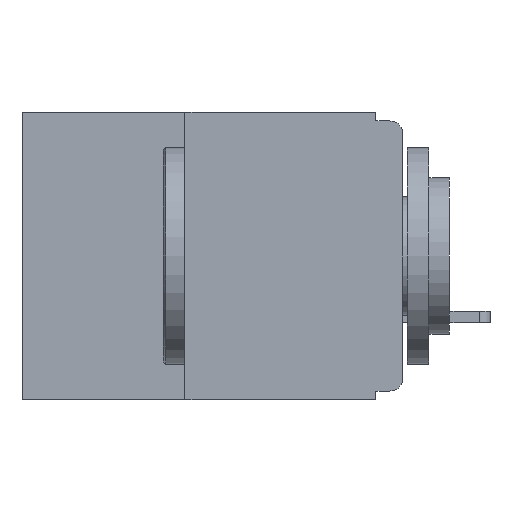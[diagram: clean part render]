
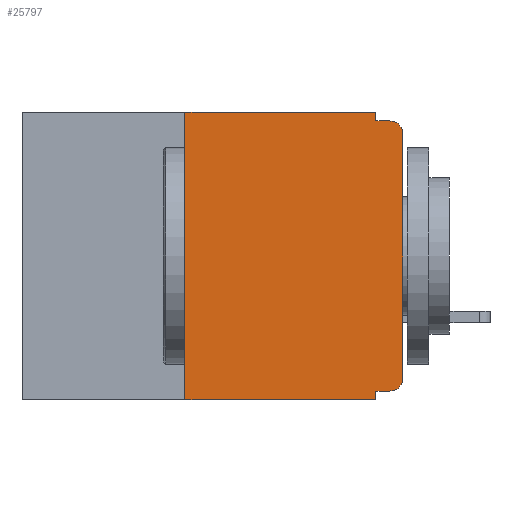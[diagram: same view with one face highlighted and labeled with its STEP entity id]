
A CAD part, left-side view. The second image highlights one B-rep face of the part: STEP entity #25797.
In plain terms, the highlighted planar face has unit normal (-1, 0, 0).
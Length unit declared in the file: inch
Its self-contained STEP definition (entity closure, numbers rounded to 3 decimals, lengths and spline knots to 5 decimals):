
#23 = CARTESIAN_POINT ( 'NONE',  ( 0., 0., -0.32 ) ) ;
#103 = DIRECTION ( 'NONE',  ( 0., -1., 0. ) ) ;
#634 = DIRECTION ( 'NONE',  ( 0., 0., -1. ) ) ;
#754 = FACE_OUTER_BOUND ( 'NONE', #24668, .T. ) ;
#768 = AXIS2_PLACEMENT_3D ( 'NONE', #10609, #28181, #13141 ) ;
#1409 = CARTESIAN_POINT ( 'NONE',  ( 0., 0.25, -0.33 ) ) ;
#1519 = ORIENTED_EDGE ( 'NONE', *, *, #18373, .F. ) ;
#1809 = CARTESIAN_POINT ( 'NONE',  ( 0., 0.031, 0. ) ) ;
#2441 = CARTESIAN_POINT ( 'NONE',  ( 0., 0.031, -0.33 ) ) ;
#2605 = PLANE ( 'NONE',  #13702 ) ;
#3797 = CARTESIAN_POINT ( 'NONE',  ( 0., 0.437, -0.33 ) ) ;
#4148 = VECTOR ( 'NONE', #22255, 39.37008 ) ;
#4818 = VERTEX_POINT ( 'NONE', #17904 ) ;
#5098 = LINE ( 'NONE', #14579, #24452 ) ;
#5212 = EDGE_CURVE ( 'NONE', #6871, #4818, #26192, .T. ) ;
#5271 = CARTESIAN_POINT ( 'NONE',  ( 0., 0.437, 0. ) ) ;
#5779 = LINE ( 'NONE', #1809, #4148 ) ;
#6827 = VERTEX_POINT ( 'NONE', #25525 ) ;
#6871 = VERTEX_POINT ( 'NONE', #13091 ) ;
#6910 = ORIENTED_EDGE ( 'NONE', *, *, #32550, .F. ) ;
#7882 = DIRECTION ( 'NONE',  ( 0., 0., -1. ) ) ;
#8579 = LINE ( 'NONE', #3797, #21163 ) ;
#8586 = VERTEX_POINT ( 'NONE', #2441 ) ;
#9328 = EDGE_CURVE ( 'NONE', #19104, #8586, #8579, .T. ) ;
#9631 = ORIENTED_EDGE ( 'NONE', *, *, #24382, .F. ) ;
#10068 = VECTOR ( 'NONE', #15318, 39.37008 ) ;
#10439 = ORIENTED_EDGE ( 'NONE', *, *, #27580, .F. ) ;
#10609 = CARTESIAN_POINT ( 'NONE',  ( 0., 0.015, -0.305 ) ) ;
#10892 = VERTEX_POINT ( 'NONE', #25152 ) ;
#10914 = LINE ( 'NONE', #23, #32439 ) ;
#11110 = VECTOR ( 'NONE', #103, 39.37008 ) ;
#11648 = DIRECTION ( 'NONE',  ( 0., 0., 1. ) ) ;
#12910 = CIRCLE ( 'NONE', #768, 0.015 ) ;
#13091 = CARTESIAN_POINT ( 'NONE',  ( 0., 0., -0.305 ) ) ;
#13141 = DIRECTION ( 'NONE',  ( 0., 0., -1. ) ) ;
#13702 = AXIS2_PLACEMENT_3D ( 'NONE', #5271, #22924, #7882 ) ;
#13821 = ORIENTED_EDGE ( 'NONE', *, *, #16783, .F. ) ;
#14011 = CARTESIAN_POINT ( 'NONE',  ( 0., 0.25, 0. ) ) ;
#14579 = CARTESIAN_POINT ( 'NONE',  ( 0., 0., -0.01 ) ) ;
#14697 = LINE ( 'NONE', #1409, #28028 ) ;
#15318 = DIRECTION ( 'NONE',  ( 0., 0., -1. ) ) ;
#16006 = DIRECTION ( 'NONE',  ( -1., 0., 0. ) ) ;
#16510 = VERTEX_POINT ( 'NONE', #14011 ) ;
#16783 = EDGE_CURVE ( 'NONE', #17514, #8586, #21857, .T. ) ;
#17514 = VERTEX_POINT ( 'NONE', #28196 ) ;
#17852 = LINE ( 'NONE', #18043, #11110 ) ;
#17904 = CARTESIAN_POINT ( 'NONE',  ( 0., 0., -0.025 ) ) ;
#17944 = CARTESIAN_POINT ( 'NONE',  ( 0., 0.25, -0.33 ) ) ;
#17963 = DIRECTION ( 'NONE',  ( 0., 1., 0. ) ) ;
#18043 = CARTESIAN_POINT ( 'NONE',  ( 0., 0.437, 0. ) ) ;
#18373 = EDGE_CURVE ( 'NONE', #19104, #16510, #14697, .T. ) ;
#19019 = DIRECTION ( 'NONE',  ( 0., -1., 0. ) ) ;
#19104 = VERTEX_POINT ( 'NONE', #17944 ) ;
#19611 = DIRECTION ( 'NONE',  ( 0., -1., 0. ) ) ;
#19684 = VERTEX_POINT ( 'NONE', #30311 ) ;
#20657 = VERTEX_POINT ( 'NONE', #25388 ) ;
#21163 = VECTOR ( 'NONE', #19019, 39.37008 ) ;
#21264 = ORIENTED_EDGE ( 'NONE', *, *, #9328, .T. ) ;
#21857 = LINE ( 'NONE', #30287, #10068 ) ;
#22099 = ORIENTED_EDGE ( 'NONE', *, *, #5212, .T. ) ;
#22110 = CIRCLE ( 'NONE', #29321, 0.015 ) ;
#22255 = DIRECTION ( 'NONE',  ( 0., 0., -1. ) ) ;
#22924 = DIRECTION ( 'NONE',  ( 1., 0., 0. ) ) ;
#24382 = EDGE_CURVE ( 'NONE', #6827, #10892, #5779, .T. ) ;
#24452 = VECTOR ( 'NONE', #19611, 39.37008 ) ;
#24493 = CARTESIAN_POINT ( 'NONE',  ( 0., 0., 0. ) ) ;
#24612 = DIRECTION ( 'NONE',  ( 0., 0., 1. ) ) ;
#24622 = EDGE_CURVE ( 'NONE', #20657, #6871, #12910, .T. ) ;
#24668 = EDGE_LOOP ( 'NONE', ( #22099, #32067, #25382, #9631, #10439, #1519, #21264, #13821, #6910, #27965 ) ) ;
#25152 = CARTESIAN_POINT ( 'NONE',  ( 0., 0.031, -0.01 ) ) ;
#25382 = ORIENTED_EDGE ( 'NONE', *, *, #28004, .F. ) ;
#25388 = CARTESIAN_POINT ( 'NONE',  ( 0., 0.015, -0.32 ) ) ;
#25525 = CARTESIAN_POINT ( 'NONE',  ( 0., 0.031, 0. ) ) ;
#25797 = ADVANCED_FACE ( 'NONE', ( #754 ), #2605, .F. ) ;
#26192 = LINE ( 'NONE', #24493, #31964 ) ;
#27580 = EDGE_CURVE ( 'NONE', #16510, #6827, #17852, .T. ) ;
#27965 = ORIENTED_EDGE ( 'NONE', *, *, #24622, .T. ) ;
#28004 = EDGE_CURVE ( 'NONE', #10892, #19684, #5098, .T. ) ;
#28028 = VECTOR ( 'NONE', #11648, 39.37008 ) ;
#28181 = DIRECTION ( 'NONE',  ( -1., 0., 0. ) ) ;
#28196 = CARTESIAN_POINT ( 'NONE',  ( 0., 0.031, -0.32 ) ) ;
#28321 = EDGE_CURVE ( 'NONE', #4818, #19684, #22110, .T. ) ;
#29321 = AXIS2_PLACEMENT_3D ( 'NONE', #30956, #16006, #634 ) ;
#30287 = CARTESIAN_POINT ( 'NONE',  ( 0., 0.031, -0.33 ) ) ;
#30311 = CARTESIAN_POINT ( 'NONE',  ( 0., 0.015, -0.01 ) ) ;
#30956 = CARTESIAN_POINT ( 'NONE',  ( 0., 0.015, -0.025 ) ) ;
#31964 = VECTOR ( 'NONE', #24612, 39.37008 ) ;
#32067 = ORIENTED_EDGE ( 'NONE', *, *, #28321, .T. ) ;
#32439 = VECTOR ( 'NONE', #17963, 39.37008 ) ;
#32550 = EDGE_CURVE ( 'NONE', #20657, #17514, #10914, .T. ) ;
